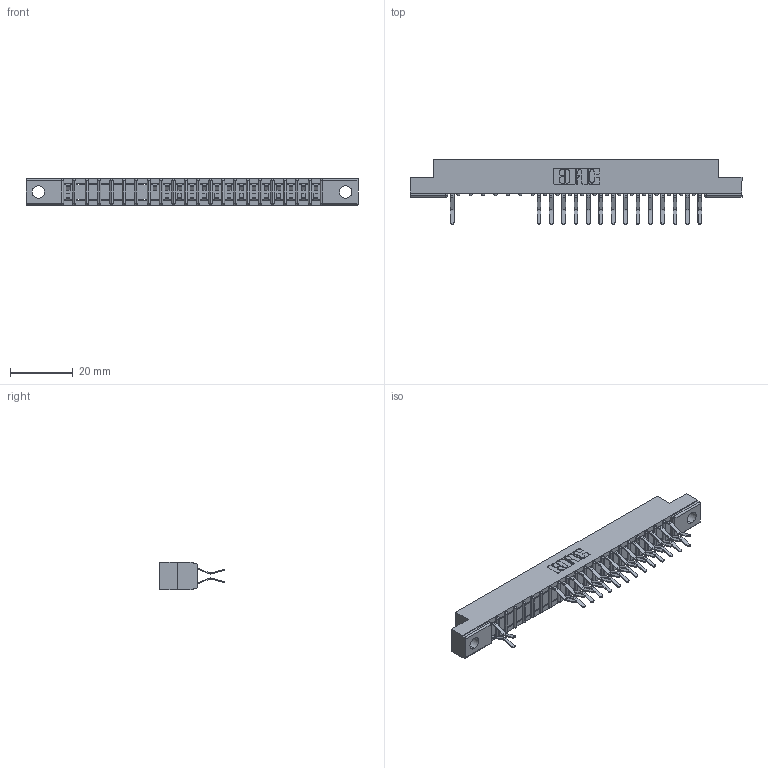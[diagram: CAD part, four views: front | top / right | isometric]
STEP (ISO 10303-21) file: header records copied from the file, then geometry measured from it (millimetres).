
FILE_DESCRIPTION (( 'STEP AP203' ), '1' );
FILE_NAME ('307-042-560-202.STEP', '2018-08-05T18:43:19', ( '' ), ( '' ), 'SwSTEP 2.0', 'SolidWorks 2016', '' );
FILE_SCHEMA (( 'CONFIG_CONTROL_DESIGN' ));
Length unit declared in the file: inch
Products named in the file (3): 307 Part_.128 Dia Mounting Holes; 307-290-001_560; 307-042-560-202
Assembly tree (30 placements, depth 2):
  307-042-560-202
    307 Part_.128 Dia Mounting Holes
    307-290-001_560  x29
Bounding box: 106.22 x 20.73 x 8.71 mm (x, y, z)
Volume: 6728.2 mm3; surface area: 10903.9 mm2
Topology: 30 solids, 30 shells, 1720 faces, 4857 edges, 3138 vertices
Faces by surface type: plane 1105, cylinder 571, sphere 44
Entity records: 20954 total; most frequent: CARTESIAN_POINT 3488, ORIENTED_EDGE 3466, DIRECTION 3413, EDGE_CURVE 1733, LINE 1319, VECTOR 1319, VERTEX_POINT 1122, AXIS2_PLACEMENT_3D 1047
